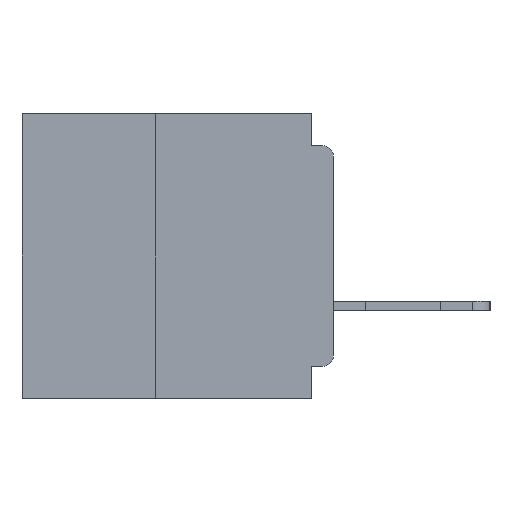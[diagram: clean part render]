
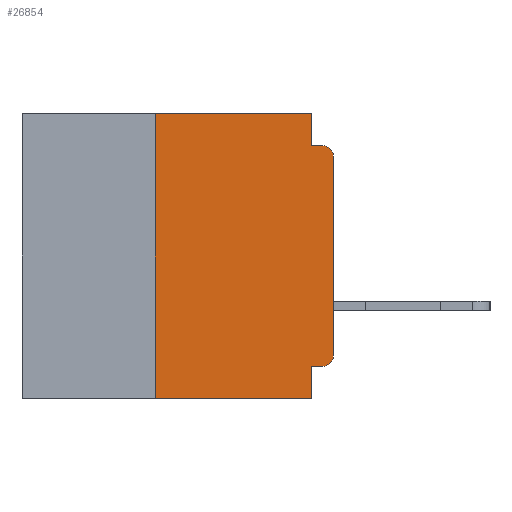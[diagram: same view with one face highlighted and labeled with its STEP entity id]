
A CAD part, left-side view. The second image highlights one B-rep face of the part: STEP entity #26854.
In plain terms, the highlighted planar face has unit normal (-1, 0, 0).
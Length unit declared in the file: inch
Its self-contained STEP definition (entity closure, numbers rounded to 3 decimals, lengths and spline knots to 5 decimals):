
#759 = FACE_OUTER_BOUND ( 'NONE', #15068, .T. ) ;
#4934 = DIRECTION ( 'NONE',  ( 1., 0., 0. ) ) ;
#5263 = VERTEX_POINT ( 'NONE', #14584 ) ;
#5722 = CARTESIAN_POINT ( 'NONE',  ( 0., 0., -0.06 ) ) ;
#6035 = ORIENTED_EDGE ( 'NONE', *, *, #44236, .F. ) ;
#6128 = VECTOR ( 'NONE', #6145, 39.37008 ) ;
#6145 = DIRECTION ( 'NONE',  ( 0., 0., -1. ) ) ;
#6384 = CARTESIAN_POINT ( 'NONE',  ( 0., 0.031, -0.4 ) ) ;
#7521 = LINE ( 'NONE', #41110, #6128 ) ;
#7827 = CARTESIAN_POINT ( 'NONE',  ( 0., 0.25, -0.4 ) ) ;
#8543 = ORIENTED_EDGE ( 'NONE', *, *, #15752, .T. ) ;
#10023 = VERTEX_POINT ( 'NONE', #41962 ) ;
#11284 = CARTESIAN_POINT ( 'NONE',  ( 0., 0.015, -0.045 ) ) ;
#12281 = DIRECTION ( 'NONE',  ( 0., 0., 1. ) ) ;
#12686 = AXIS2_PLACEMENT_3D ( 'NONE', #42210, #15919, #46626 ) ;
#13164 = VERTEX_POINT ( 'NONE', #19652 ) ;
#13642 = CARTESIAN_POINT ( 'NONE',  ( 0., 0.437, 0. ) ) ;
#14584 = CARTESIAN_POINT ( 'NONE',  ( 0., 0.25, -0.4 ) ) ;
#15054 = CIRCLE ( 'NONE', #12686, 0.015 ) ;
#15068 = EDGE_LOOP ( 'NONE', ( #41092, #8543, #20072, #19754, #16167, #23811, #25828, #6035, #18772, #39885 ) ) ;
#15069 = EDGE_CURVE ( 'NONE', #21304, #23577, #48703, .T. ) ;
#15752 = EDGE_CURVE ( 'NONE', #53998, #23577, #15054, .T. ) ;
#15919 = DIRECTION ( 'NONE',  ( -1., 0., 0. ) ) ;
#16167 = ORIENTED_EDGE ( 'NONE', *, *, #36842, .F. ) ;
#16750 = VERTEX_POINT ( 'NONE', #50017 ) ;
#17190 = LINE ( 'NONE', #39949, #41912 ) ;
#18294 = CARTESIAN_POINT ( 'NONE',  ( 0., 0.031, -0.4 ) ) ;
#18331 = LINE ( 'NONE', #18294, #34782 ) ;
#18772 = ORIENTED_EDGE ( 'NONE', *, *, #18859, .F. ) ;
#18859 = EDGE_CURVE ( 'NONE', #38720, #13164, #45014, .T. ) ;
#19238 = DIRECTION ( 'NONE',  ( 0., -1., 0. ) ) ;
#19652 = CARTESIAN_POINT ( 'NONE',  ( 0., 0.031, -0.355 ) ) ;
#19653 = VERTEX_POINT ( 'NONE', #44445 ) ;
#19754 = ORIENTED_EDGE ( 'NONE', *, *, #21807, .F. ) ;
#20072 = ORIENTED_EDGE ( 'NONE', *, *, #15069, .F. ) ;
#20157 = DIRECTION ( 'NONE',  ( -1., 0., 0. ) ) ;
#21304 = VERTEX_POINT ( 'NONE', #29069 ) ;
#21661 = VECTOR ( 'NONE', #39198, 39.37008 ) ;
#21807 = EDGE_CURVE ( 'NONE', #16750, #21304, #7521, .T. ) ;
#22723 = DIRECTION ( 'NONE',  ( 0., 0., -1. ) ) ;
#23577 = VERTEX_POINT ( 'NONE', #11284 ) ;
#23811 = ORIENTED_EDGE ( 'NONE', *, *, #50648, .F. ) ;
#25637 = AXIS2_PLACEMENT_3D ( 'NONE', #13642, #4934, #35698 ) ;
#25828 = ORIENTED_EDGE ( 'NONE', *, *, #27885, .T. ) ;
#26048 = VECTOR ( 'NONE', #35475, 39.37008 ) ;
#26653 = EDGE_CURVE ( 'NONE', #38720, #10023, #48183, .T. ) ;
#26854 = ADVANCED_FACE ( 'NONE', ( #759 ), #53187, .F. ) ;
#26919 = DIRECTION ( 'NONE',  ( 0., -1., 0. ) ) ;
#27860 = CARTESIAN_POINT ( 'NONE',  ( 0., 0., -0.045 ) ) ;
#27885 = EDGE_CURVE ( 'NONE', #5263, #36440, #39078, .T. ) ;
#29069 = CARTESIAN_POINT ( 'NONE',  ( 0., 0.031, -0.045 ) ) ;
#29660 = AXIS2_PLACEMENT_3D ( 'NONE', #46458, #20157, #50895 ) ;
#30962 = CARTESIAN_POINT ( 'NONE',  ( 0., 0.015, -0.355 ) ) ;
#32025 = CARTESIAN_POINT ( 'NONE',  ( 0., 0., 0. ) ) ;
#32671 = VECTOR ( 'NONE', #36405, 39.37008 ) ;
#34782 = VECTOR ( 'NONE', #22723, 39.37008 ) ;
#35475 = DIRECTION ( 'NONE',  ( 0., -1., 0. ) ) ;
#35698 = DIRECTION ( 'NONE',  ( 0., 0., -1. ) ) ;
#36405 = DIRECTION ( 'NONE',  ( 0., 0., 1. ) ) ;
#36440 = VERTEX_POINT ( 'NONE', #6384 ) ;
#36597 = VECTOR ( 'NONE', #12281, 39.37008 ) ;
#36842 = EDGE_CURVE ( 'NONE', #19653, #16750, #17190, .T. ) ;
#37980 = LINE ( 'NONE', #7827, #36597 ) ;
#38720 = VERTEX_POINT ( 'NONE', #30962 ) ;
#39078 = LINE ( 'NONE', #44337, #26048 ) ;
#39198 = DIRECTION ( 'NONE',  ( 0., 1., 0. ) ) ;
#39885 = ORIENTED_EDGE ( 'NONE', *, *, #26653, .T. ) ;
#39949 = CARTESIAN_POINT ( 'NONE',  ( 0., 0.437, 0. ) ) ;
#41092 = ORIENTED_EDGE ( 'NONE', *, *, #54618, .T. ) ;
#41110 = CARTESIAN_POINT ( 'NONE',  ( 0., 0.031, 0. ) ) ;
#41912 = VECTOR ( 'NONE', #26919, 39.37008 ) ;
#41962 = CARTESIAN_POINT ( 'NONE',  ( 0., 0., -0.34 ) ) ;
#42210 = CARTESIAN_POINT ( 'NONE',  ( 0., 0.015, -0.06 ) ) ;
#43644 = CARTESIAN_POINT ( 'NONE',  ( 0., 0., -0.355 ) ) ;
#44236 = EDGE_CURVE ( 'NONE', #13164, #36440, #18331, .T. ) ;
#44337 = CARTESIAN_POINT ( 'NONE',  ( 0., 0.437, -0.4 ) ) ;
#44370 = LINE ( 'NONE', #32025, #32671 ) ;
#44445 = CARTESIAN_POINT ( 'NONE',  ( 0., 0.25, 0. ) ) ;
#45014 = LINE ( 'NONE', #43644, #21661 ) ;
#46458 = CARTESIAN_POINT ( 'NONE',  ( 0., 0.015, -0.34 ) ) ;
#46626 = DIRECTION ( 'NONE',  ( 0., 0., -1. ) ) ;
#47303 = VECTOR ( 'NONE', #19238, 39.37008 ) ;
#48183 = CIRCLE ( 'NONE', #29660, 0.015 ) ;
#48703 = LINE ( 'NONE', #27860, #47303 ) ;
#50017 = CARTESIAN_POINT ( 'NONE',  ( 0., 0.031, 0. ) ) ;
#50648 = EDGE_CURVE ( 'NONE', #5263, #19653, #37980, .T. ) ;
#50895 = DIRECTION ( 'NONE',  ( 0., 0., -1. ) ) ;
#53187 = PLANE ( 'NONE',  #25637 ) ;
#53998 = VERTEX_POINT ( 'NONE', #5722 ) ;
#54618 = EDGE_CURVE ( 'NONE', #10023, #53998, #44370, .T. ) ;
